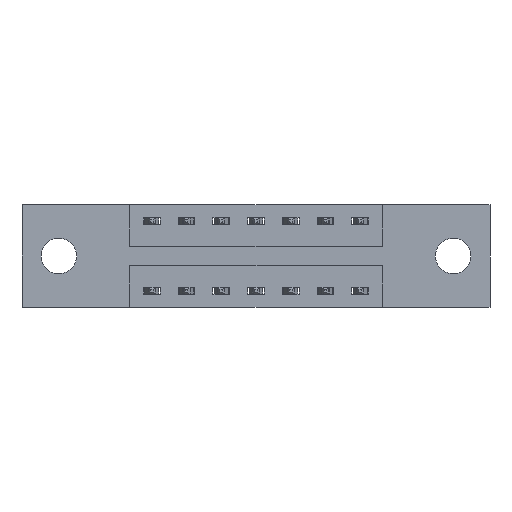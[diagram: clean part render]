
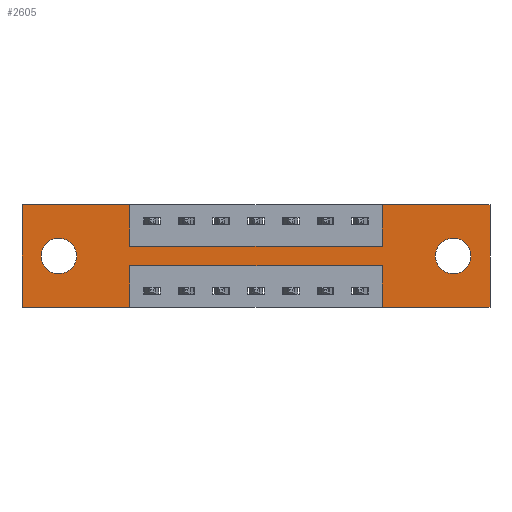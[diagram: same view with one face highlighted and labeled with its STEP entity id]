
A CAD part, front view. The second image highlights one B-rep face of the part: STEP entity #2605.
In plain terms, the highlighted planar face has unit normal (0, -1, 0).
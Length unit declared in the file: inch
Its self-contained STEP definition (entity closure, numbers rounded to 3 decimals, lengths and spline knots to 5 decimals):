
#1 = VERTEX_POINT ( 'NONE', #3922 ) ;
#18 = AXIS2_PLACEMENT_3D ( 'NONE', #9059, #5593, #1167 ) ;
#28 = ORIENTED_EDGE ( 'NONE', *, *, #6222, .F. ) ;
#168 = AXIS2_PLACEMENT_3D ( 'NONE', #9166, #6357, #7032 ) ;
#200 = ORIENTED_EDGE ( 'NONE', *, *, #3746, .T. ) ;
#227 = CARTESIAN_POINT ( 'NONE',  ( 1.5525, 0., -0.121 ) ) ;
#256 = VERTEX_POINT ( 'NONE', #2040 ) ;
#309 = DIRECTION ( 'NONE',  ( 0., 1., 0. ) ) ;
#406 = PLANE ( 'NONE',  #18 ) ;
#509 = ORIENTED_EDGE ( 'NONE', *, *, #5627, .T. ) ;
#555 = VERTEX_POINT ( 'NONE', #1945 ) ;
#800 = DIRECTION ( 'NONE',  ( 1., 0., 0. ) ) ;
#905 = DIRECTION ( 'NONE',  ( 1., 0., 0. ) ) ;
#915 = FACE_BOUND ( 'NONE', #2802, .T. ) ;
#1046 = ORIENTED_EDGE ( 'NONE', *, *, #5009, .F. ) ;
#1119 = LINE ( 'NONE', #7997, #6777 ) ;
#1167 = DIRECTION ( 'NONE',  ( 0., 0., -1. ) ) ;
#1193 = CARTESIAN_POINT ( 'NONE',  ( 0., 0., -0.37 ) ) ;
#1195 = VERTEX_POINT ( 'NONE', #3075 ) ;
#1322 = ORIENTED_EDGE ( 'NONE', *, *, #3382, .F. ) ;
#1507 = VERTEX_POINT ( 'NONE', #227 ) ;
#1550 = CARTESIAN_POINT ( 'NONE',  ( 0., 0., 0. ) ) ;
#1664 = VECTOR ( 'NONE', #7564, 39.37008 ) ;
#1887 = AXIS2_PLACEMENT_3D ( 'NONE', #6678, #2253, #7385 ) ;
#1945 = CARTESIAN_POINT ( 'NONE',  ( 0.3875, 0., -0.22 ) ) ;
#2040 = CARTESIAN_POINT ( 'NONE',  ( 0.3875, 0., 0. ) ) ;
#2049 = ORIENTED_EDGE ( 'NONE', *, *, #6322, .F. ) ;
#2069 = EDGE_CURVE ( 'NONE', #1, #1507, #3198, .T. ) ;
#2105 = ORIENTED_EDGE ( 'NONE', *, *, #2069, .T. ) ;
#2201 = DIRECTION ( 'NONE',  ( 0., 0., 1. ) ) ;
#2209 = ORIENTED_EDGE ( 'NONE', *, *, #5948, .F. ) ;
#2253 = DIRECTION ( 'NONE',  ( 0., 1., 0. ) ) ;
#2277 = VERTEX_POINT ( 'NONE', #3169 ) ;
#2370 = CARTESIAN_POINT ( 'NONE',  ( 0., 0., -0.37 ) ) ;
#2485 = EDGE_LOOP ( 'NONE', ( #1046, #7599, #6462, #7824, #28, #7359, #1322, #6963, #8301, #5526, #2049, #2209 ) ) ;
#2605 = ADVANCED_FACE ( 'NONE', ( #8600, #915, #4932 ), #406, .T. ) ;
#2802 = EDGE_LOOP ( 'NONE', ( #6253, #200 ) ) ;
#2806 = VERTEX_POINT ( 'NONE', #5399 ) ;
#2829 = LINE ( 'NONE', #6421, #6561 ) ;
#2840 = CARTESIAN_POINT ( 'NONE',  ( 0.3875, 0., -0.37 ) ) ;
#3018 = CARTESIAN_POINT ( 'NONE',  ( 0.1325, 0., -0.249 ) ) ;
#3075 = CARTESIAN_POINT ( 'NONE',  ( 0.1325, 0., -0.121 ) ) ;
#3107 = VERTEX_POINT ( 'NONE', #3018 ) ;
#3134 = CARTESIAN_POINT ( 'NONE',  ( 1.2975, 0., -0.37 ) ) ;
#3154 = CIRCLE ( 'NONE', #5403, 0.064 ) ;
#3169 = CARTESIAN_POINT ( 'NONE',  ( 0.3875, 0., -0.37 ) ) ;
#3198 = CIRCLE ( 'NONE', #168, 0.064 ) ;
#3382 = EDGE_CURVE ( 'NONE', #7573, #5205, #3539, .T. ) ;
#3488 = EDGE_CURVE ( 'NONE', #5098, #6105, #9281, .T. ) ;
#3536 = CARTESIAN_POINT ( 'NONE',  ( 1.5525, 0., -0.185 ) ) ;
#3539 = LINE ( 'NONE', #6619, #5546 ) ;
#3561 = DIRECTION ( 'NONE',  ( 0., 0., 1. ) ) ;
#3566 = LINE ( 'NONE', #7401, #5146 ) ;
#3622 = DIRECTION ( 'NONE',  ( 0., 0., -1. ) ) ;
#3746 = EDGE_CURVE ( 'NONE', #3107, #1195, #3154, .T. ) ;
#3922 = CARTESIAN_POINT ( 'NONE',  ( 1.5525, 0., -0.249 ) ) ;
#4071 = VERTEX_POINT ( 'NONE', #5395 ) ;
#4098 = CARTESIAN_POINT ( 'NONE',  ( 1.2975, 0., -0.22 ) ) ;
#4157 = EDGE_LOOP ( 'NONE', ( #509, #2105 ) ) ;
#4361 = DIRECTION ( 'NONE',  ( 0., 0., -1. ) ) ;
#4554 = VERTEX_POINT ( 'NONE', #6223 ) ;
#4557 = CARTESIAN_POINT ( 'NONE',  ( 1.2975, 0., -0.37 ) ) ;
#4566 = EDGE_CURVE ( 'NONE', #6105, #555, #5928, .T. ) ;
#4816 = CARTESIAN_POINT ( 'NONE',  ( 0.1325, 0., -0.185 ) ) ;
#4931 = LINE ( 'NONE', #1550, #6571 ) ;
#4932 = FACE_OUTER_BOUND ( 'NONE', #2485, .T. ) ;
#4946 = VECTOR ( 'NONE', #3622, 39.37008 ) ;
#5009 = EDGE_CURVE ( 'NONE', #555, #2277, #5162, .T. ) ;
#5086 = EDGE_CURVE ( 'NONE', #1195, #3107, #5920, .T. ) ;
#5098 = VERTEX_POINT ( 'NONE', #4557 ) ;
#5146 = VECTOR ( 'NONE', #800, 39.37008 ) ;
#5162 = LINE ( 'NONE', #2840, #4946 ) ;
#5205 = VERTEX_POINT ( 'NONE', #6812 ) ;
#5395 = CARTESIAN_POINT ( 'NONE',  ( 0., 0., 0. ) ) ;
#5399 = CARTESIAN_POINT ( 'NONE',  ( 0.3875, 0., -0.15 ) ) ;
#5403 = AXIS2_PLACEMENT_3D ( 'NONE', #4816, #309, #5519 ) ;
#5500 = VECTOR ( 'NONE', #8305, 39.37008 ) ;
#5517 = VERTEX_POINT ( 'NONE', #1193 ) ;
#5519 = DIRECTION ( 'NONE',  ( 0., 0., 1. ) ) ;
#5526 = ORIENTED_EDGE ( 'NONE', *, *, #5828, .F. ) ;
#5538 = VERTEX_POINT ( 'NONE', #8424 ) ;
#5546 = VECTOR ( 'NONE', #2201, 39.37008 ) ;
#5593 = DIRECTION ( 'NONE',  ( 0., -1., 0. ) ) ;
#5627 = EDGE_CURVE ( 'NONE', #1507, #1, #8706, .T. ) ;
#5671 = DIRECTION ( 'NONE',  ( -1., 0., 0. ) ) ;
#5786 = EDGE_CURVE ( 'NONE', #5205, #4554, #3566, .T. ) ;
#5828 = EDGE_CURVE ( 'NONE', #4071, #256, #4931, .T. ) ;
#5920 = CIRCLE ( 'NONE', #1887, 0.064 ) ;
#5928 = LINE ( 'NONE', #7618, #5500 ) ;
#5948 = EDGE_CURVE ( 'NONE', #2277, #5517, #7551, .T. ) ;
#6056 = CARTESIAN_POINT ( 'NONE',  ( 0.3875, 0., -0.15 ) ) ;
#6105 = VERTEX_POINT ( 'NONE', #4098 ) ;
#6211 = EDGE_CURVE ( 'NONE', #5538, #5098, #7014, .T. ) ;
#6222 = EDGE_CURVE ( 'NONE', #4554, #5538, #2829, .T. ) ;
#6223 = CARTESIAN_POINT ( 'NONE',  ( 1.685, 0., 0. ) ) ;
#6253 = ORIENTED_EDGE ( 'NONE', *, *, #5086, .T. ) ;
#6322 = EDGE_CURVE ( 'NONE', #5517, #4071, #7752, .T. ) ;
#6357 = DIRECTION ( 'NONE',  ( 0., 1., 0. ) ) ;
#6421 = CARTESIAN_POINT ( 'NONE',  ( 1.685, 0., 0. ) ) ;
#6462 = ORIENTED_EDGE ( 'NONE', *, *, #3488, .F. ) ;
#6561 = VECTOR ( 'NONE', #7132, 39.37008 ) ;
#6571 = VECTOR ( 'NONE', #6735, 39.37008 ) ;
#6619 = CARTESIAN_POINT ( 'NONE',  ( 1.2975, 0., 0. ) ) ;
#6678 = CARTESIAN_POINT ( 'NONE',  ( 0.1325, 0., -0.185 ) ) ;
#6735 = DIRECTION ( 'NONE',  ( 1., 0., 0. ) ) ;
#6777 = VECTOR ( 'NONE', #8669, 39.37008 ) ;
#6812 = CARTESIAN_POINT ( 'NONE',  ( 1.2975, 0., 0. ) ) ;
#6963 = ORIENTED_EDGE ( 'NONE', *, *, #8415, .F. ) ;
#7014 = LINE ( 'NONE', #7100, #8589 ) ;
#7032 = DIRECTION ( 'NONE',  ( 0., 0., -1. ) ) ;
#7100 = CARTESIAN_POINT ( 'NONE',  ( 0., 0., -0.37 ) ) ;
#7102 = VECTOR ( 'NONE', #905, 39.37008 ) ;
#7132 = DIRECTION ( 'NONE',  ( 0., 0., -1. ) ) ;
#7312 = AXIS2_PLACEMENT_3D ( 'NONE', #3536, #8541, #4361 ) ;
#7359 = ORIENTED_EDGE ( 'NONE', *, *, #5786, .F. ) ;
#7385 = DIRECTION ( 'NONE',  ( 0., 0., 1. ) ) ;
#7401 = CARTESIAN_POINT ( 'NONE',  ( 0., 0., 0. ) ) ;
#7539 = VECTOR ( 'NONE', #3561, 39.37008 ) ;
#7551 = LINE ( 'NONE', #2370, #9118 ) ;
#7564 = DIRECTION ( 'NONE',  ( 0., 0., 1. ) ) ;
#7573 = VERTEX_POINT ( 'NONE', #7593 ) ;
#7593 = CARTESIAN_POINT ( 'NONE',  ( 1.2975, 0., -0.15 ) ) ;
#7599 = ORIENTED_EDGE ( 'NONE', *, *, #4566, .F. ) ;
#7618 = CARTESIAN_POINT ( 'NONE',  ( 0.3875, 0., -0.22 ) ) ;
#7752 = LINE ( 'NONE', #8499, #7539 ) ;
#7824 = ORIENTED_EDGE ( 'NONE', *, *, #6211, .F. ) ;
#7997 = CARTESIAN_POINT ( 'NONE',  ( 0.3875, 0., 0. ) ) ;
#8168 = EDGE_CURVE ( 'NONE', #256, #2806, #1119, .T. ) ;
#8301 = ORIENTED_EDGE ( 'NONE', *, *, #8168, .F. ) ;
#8305 = DIRECTION ( 'NONE',  ( -1., 0., 0. ) ) ;
#8415 = EDGE_CURVE ( 'NONE', #2806, #7573, #8888, .T. ) ;
#8424 = CARTESIAN_POINT ( 'NONE',  ( 1.685, 0., -0.37 ) ) ;
#8499 = CARTESIAN_POINT ( 'NONE',  ( 0., 0., 0. ) ) ;
#8541 = DIRECTION ( 'NONE',  ( 0., 1., 0. ) ) ;
#8589 = VECTOR ( 'NONE', #5671, 39.37008 ) ;
#8600 = FACE_BOUND ( 'NONE', #4157, .T. ) ;
#8669 = DIRECTION ( 'NONE',  ( 0., 0., -1. ) ) ;
#8706 = CIRCLE ( 'NONE', #7312, 0.064 ) ;
#8871 = DIRECTION ( 'NONE',  ( -1., 0., 0. ) ) ;
#8888 = LINE ( 'NONE', #6056, #7102 ) ;
#9059 = CARTESIAN_POINT ( 'NONE',  ( 0., 0., -0.37 ) ) ;
#9118 = VECTOR ( 'NONE', #8871, 39.37008 ) ;
#9166 = CARTESIAN_POINT ( 'NONE',  ( 1.5525, 0., -0.185 ) ) ;
#9281 = LINE ( 'NONE', #3134, #1664 ) ;
